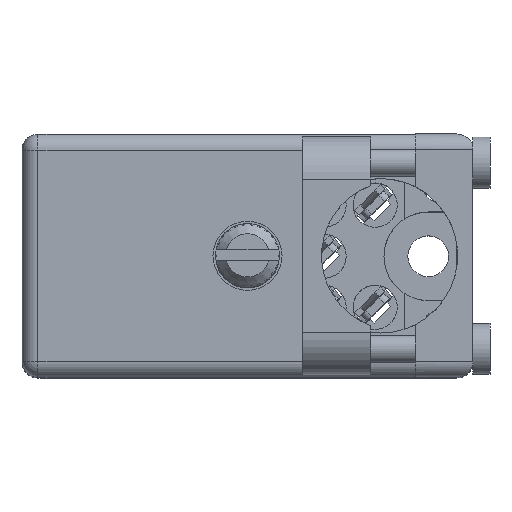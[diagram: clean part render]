
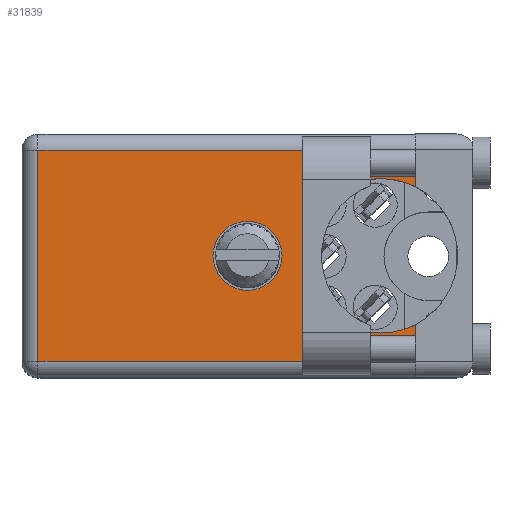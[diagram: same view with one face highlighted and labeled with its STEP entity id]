
A CAD part, top view. The second image highlights one B-rep face of the part: STEP entity #31839.
In plain terms, the highlighted face is planar.
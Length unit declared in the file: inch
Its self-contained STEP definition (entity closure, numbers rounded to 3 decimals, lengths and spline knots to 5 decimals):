
#1441 = CARTESIAN_POINT ( 'NONE',  ( 1.053, 0.906, -0.3575 ) ) ;
#1453 = EDGE_CURVE ( 'NONE', #167879, #76739, #99273, .T. ) ;
#2789 = VERTEX_POINT ( 'NONE', #125294 ) ;
#4079 = DIRECTION ( 'NONE',  ( 0., 0., 1. ) ) ;
#6087 = CARTESIAN_POINT ( 'NONE',  ( 0.6625, 0.906, -0.3575 ) ) ;
#6642 = CARTESIAN_POINT ( 'NONE',  ( 1.053, 0.906, -0.1305 ) ) ;
#8615 = EDGE_CURVE ( 'NONE', #175801, #86376, #179440, .T. ) ;
#21017 = VECTOR ( 'NONE', #139346, 39.37008 ) ;
#21289 = ORIENTED_EDGE ( 'NONE', *, *, #150255, .T. ) ;
#21978 = ORIENTED_EDGE ( 'NONE', *, *, #8615, .F. ) ;
#26498 = CARTESIAN_POINT ( 'NONE',  ( 0.047, 0.906, -0.047 ) ) ;
#26983 = CARTESIAN_POINT ( 'NONE',  ( 0.047, 0.906, -0.715 ) ) ;
#27030 = AXIS2_PLACEMENT_3D ( 'NONE', #6087, #137686, #178063 ) ;
#27298 = CIRCLE ( 'NONE', #105169, 0.227 ) ;
#28996 = VERTEX_POINT ( 'NONE', #66815 ) ;
#31839 = ADVANCED_FACE ( 'NONE', ( #140889, #69459 ), #142707, .T. ) ;
#32128 = EDGE_CURVE ( 'NONE', #162079, #37588, #56029, .T. ) ;
#33896 = ORIENTED_EDGE ( 'NONE', *, *, #143700, .F. ) ;
#36815 = LINE ( 'NONE', #151505, #114211 ) ;
#37588 = VERTEX_POINT ( 'NONE', #141387 ) ;
#37963 = CARTESIAN_POINT ( 'NONE',  ( 1.053, 0.906, -0.3575 ) ) ;
#39135 = CIRCLE ( 'NONE', #27030, 0.1015 ) ;
#40752 = VECTOR ( 'NONE', #141680, 39.37008 ) ;
#47067 = DIRECTION ( 'NONE',  ( 1., 0., 0. ) ) ;
#49238 = LINE ( 'NONE', #86161, #112307 ) ;
#54733 = CARTESIAN_POINT ( 'NONE',  ( 1.155, 0.906, 0. ) ) ;
#56001 = CARTESIAN_POINT ( 'NONE',  ( 0.6625, 0.906, -0.256 ) ) ;
#56029 = CIRCLE ( 'NONE', #167100, 0.1015 ) ;
#56972 = DIRECTION ( 'NONE',  ( 0., 0., 1. ) ) ;
#58955 = AXIS2_PLACEMENT_3D ( 'NONE', #184061, #141806, #127654 ) ;
#62143 = ORIENTED_EDGE ( 'NONE', *, *, #180424, .F. ) ;
#66815 = CARTESIAN_POINT ( 'NONE',  ( 1.155, 0.906, -0.15471 ) ) ;
#68265 = CIRCLE ( 'NONE', #74239, 0.227 ) ;
#69459 = FACE_BOUND ( 'NONE', #115500, .T. ) ;
#72192 = CARTESIAN_POINT ( 'NONE',  ( 0.6625, 0.906, -0.3575 ) ) ;
#74239 = AXIS2_PLACEMENT_3D ( 'NONE', #144193, #90480, #4079 ) ;
#76739 = VERTEX_POINT ( 'NONE', #26498 ) ;
#77423 = DIRECTION ( 'NONE',  ( 0., 1., 0. ) ) ;
#86161 = CARTESIAN_POINT ( 'NONE',  ( 0., 0.906, -0.668 ) ) ;
#86376 = VERTEX_POINT ( 'NONE', #6642 ) ;
#90205 = CARTESIAN_POINT ( 'NONE',  ( 1.155, 0.906, -0.047 ) ) ;
#90480 = DIRECTION ( 'NONE',  ( 0., 1., 0. ) ) ;
#93686 = EDGE_CURVE ( 'NONE', #2789, #175801, #27298, .T. ) ;
#95298 = AXIS2_PLACEMENT_3D ( 'NONE', #37963, #77423, #134790 ) ;
#99273 = LINE ( 'NONE', #26983, #40752 ) ;
#102603 = ORIENTED_EDGE ( 'NONE', *, *, #124288, .T. ) ;
#105169 = AXIS2_PLACEMENT_3D ( 'NONE', #1441, #143432, #56972 ) ;
#112307 = VECTOR ( 'NONE', #114369, 39.37008 ) ;
#114211 = VECTOR ( 'NONE', #137373, 39.37008 ) ;
#114369 = DIRECTION ( 'NONE',  ( -1., 0., 0. ) ) ;
#115500 = EDGE_LOOP ( 'NONE', ( #133870, #33896 ) ) ;
#120287 = LINE ( 'NONE', #90205, #153055 ) ;
#124288 = EDGE_CURVE ( 'NONE', #168246, #167879, #49238, .T. ) ;
#125294 = CARTESIAN_POINT ( 'NONE',  ( 1.155, 0.906, -0.56029 ) ) ;
#127654 = DIRECTION ( 'NONE',  ( 0., 0., 1. ) ) ;
#129500 = DIRECTION ( 'NONE',  ( 0., 1., 0. ) ) ;
#130457 = EDGE_CURVE ( 'NONE', #86376, #28996, #68265, .T. ) ;
#133361 = CARTESIAN_POINT ( 'NONE',  ( 0.047, 0.906, -0.668 ) ) ;
#133870 = ORIENTED_EDGE ( 'NONE', *, *, #32128, .F. ) ;
#134790 = DIRECTION ( 'NONE',  ( 0., 0., 1. ) ) ;
#136066 = ORIENTED_EDGE ( 'NONE', *, *, #1453, .T. ) ;
#137373 = DIRECTION ( 'NONE',  ( 0., 0., 1. ) ) ;
#137686 = DIRECTION ( 'NONE',  ( 0., 1., 0. ) ) ;
#139346 = DIRECTION ( 'NONE',  ( 0., 0., 1. ) ) ;
#140889 = FACE_OUTER_BOUND ( 'NONE', #172230, .T. ) ;
#141387 = CARTESIAN_POINT ( 'NONE',  ( 0.6625, 0.906, -0.459 ) ) ;
#141680 = DIRECTION ( 'NONE',  ( 0., 0., 1. ) ) ;
#141806 = DIRECTION ( 'NONE',  ( 0., 1., 0. ) ) ;
#142707 = PLANE ( 'NONE',  #58955 ) ;
#143432 = DIRECTION ( 'NONE',  ( 0., 1., 0. ) ) ;
#143700 = EDGE_CURVE ( 'NONE', #37588, #162079, #39135, .T. ) ;
#144193 = CARTESIAN_POINT ( 'NONE',  ( 1.053, 0.906, -0.3575 ) ) ;
#145451 = ORIENTED_EDGE ( 'NONE', *, *, #145954, .F. ) ;
#145954 = EDGE_CURVE ( 'NONE', #28996, #169207, #36815, .T. ) ;
#147452 = ORIENTED_EDGE ( 'NONE', *, *, #130457, .F. ) ;
#149046 = ORIENTED_EDGE ( 'NONE', *, *, #93686, .F. ) ;
#150143 = DIRECTION ( 'NONE',  ( 0., 0., 1. ) ) ;
#150255 = EDGE_CURVE ( 'NONE', #76739, #169207, #120287, .T. ) ;
#151505 = CARTESIAN_POINT ( 'NONE',  ( 1.155, 0.906, 0. ) ) ;
#153055 = VECTOR ( 'NONE', #47067, 39.37008 ) ;
#161619 = CARTESIAN_POINT ( 'NONE',  ( 1.155, 0.906, -0.047 ) ) ;
#162079 = VERTEX_POINT ( 'NONE', #56001 ) ;
#167100 = AXIS2_PLACEMENT_3D ( 'NONE', #72192, #129500, #150143 ) ;
#167879 = VERTEX_POINT ( 'NONE', #133361 ) ;
#168246 = VERTEX_POINT ( 'NONE', #169427 ) ;
#169207 = VERTEX_POINT ( 'NONE', #161619 ) ;
#169427 = CARTESIAN_POINT ( 'NONE',  ( 1.155, 0.906, -0.668 ) ) ;
#172230 = EDGE_LOOP ( 'NONE', ( #62143, #102603, #136066, #21289, #145451, #147452, #21978, #149046 ) ) ;
#175801 = VERTEX_POINT ( 'NONE', #180710 ) ;
#178063 = DIRECTION ( 'NONE',  ( 0., 0., 1. ) ) ;
#179440 = CIRCLE ( 'NONE', #95298, 0.227 ) ;
#180424 = EDGE_CURVE ( 'NONE', #168246, #2789, #184353, .T. ) ;
#180710 = CARTESIAN_POINT ( 'NONE',  ( 1.053, 0.906, -0.5845 ) ) ;
#184061 = CARTESIAN_POINT ( 'NONE',  ( 0., 0.906, -0.715 ) ) ;
#184353 = LINE ( 'NONE', #54733, #21017 ) ;
